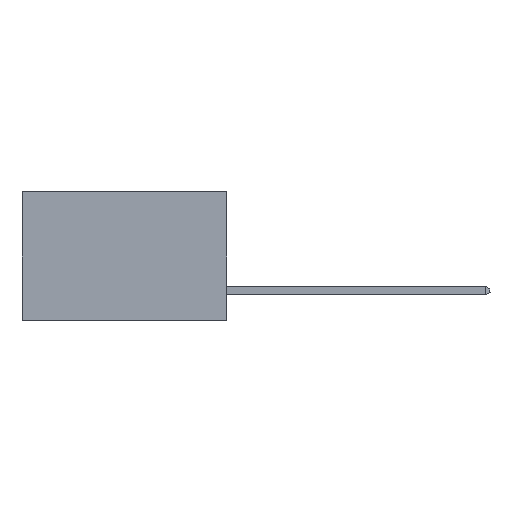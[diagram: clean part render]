
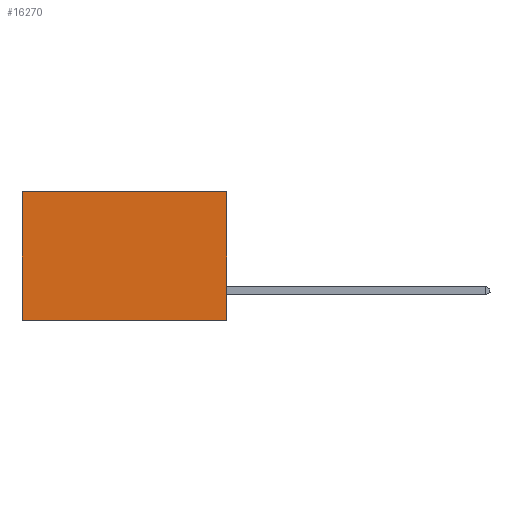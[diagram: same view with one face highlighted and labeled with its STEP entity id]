
A CAD part, left-side view. The second image highlights one B-rep face of the part: STEP entity #16270.
In plain terms, the highlighted planar face has unit normal (-1, 0, 0).
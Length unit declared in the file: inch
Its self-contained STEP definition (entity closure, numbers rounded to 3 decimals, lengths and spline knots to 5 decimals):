
#533 = VERTEX_POINT ( 'NONE', #3240 ) ;
#627 = FACE_OUTER_BOUND ( 'NONE', #21544, .T. ) ;
#714 = EDGE_CURVE ( 'NONE', #16950, #11298, #19438, .T. ) ;
#1269 = DIRECTION ( 'NONE',  ( 0., 0., -1. ) ) ;
#2451 = DIRECTION ( 'NONE',  ( 0., 1., 0. ) ) ;
#3240 = CARTESIAN_POINT ( 'NONE',  ( 0.277, 0.59, 0. ) ) ;
#4111 = CARTESIAN_POINT ( 'NONE',  ( 0.277, 0., -0.37 ) ) ;
#5904 = DIRECTION ( 'NONE',  ( 1., 0., 0. ) ) ;
#6720 = CARTESIAN_POINT ( 'NONE',  ( 0.277, 0., 0. ) ) ;
#7250 = CARTESIAN_POINT ( 'NONE',  ( 0.277, 0., -0.37 ) ) ;
#8171 = ORIENTED_EDGE ( 'NONE', *, *, #14453, .F. ) ;
#9610 = EDGE_CURVE ( 'NONE', #16950, #533, #18718, .T. ) ;
#9711 = CARTESIAN_POINT ( 'NONE',  ( 0.277, 0., -0.37 ) ) ;
#9885 = VECTOR ( 'NONE', #1269, 39.37008 ) ;
#10348 = ORIENTED_EDGE ( 'NONE', *, *, #9610, .T. ) ;
#11298 = VERTEX_POINT ( 'NONE', #15317 ) ;
#12058 = VECTOR ( 'NONE', #2451, 39.37008 ) ;
#12120 = ORIENTED_EDGE ( 'NONE', *, *, #22434, .T. ) ;
#12194 = VECTOR ( 'NONE', #15052, 39.37008 ) ;
#13154 = CARTESIAN_POINT ( 'NONE',  ( 0.277, 0., 0. ) ) ;
#13283 = CARTESIAN_POINT ( 'NONE',  ( 0.277, 0.59, -0.37 ) ) ;
#14453 = EDGE_CURVE ( 'NONE', #11298, #17278, #22154, .T. ) ;
#14880 = PLANE ( 'NONE',  #17425 ) ;
#15052 = DIRECTION ( 'NONE',  ( 0., 0., -1. ) ) ;
#15317 = CARTESIAN_POINT ( 'NONE',  ( 0.277, 0., -0.37 ) ) ;
#16270 = ADVANCED_FACE ( 'NONE', ( #627 ), #14880, .F. ) ;
#16626 = CARTESIAN_POINT ( 'NONE',  ( 0.277, 0.59, -0.37 ) ) ;
#16950 = VERTEX_POINT ( 'NONE', #13154 ) ;
#17278 = VERTEX_POINT ( 'NONE', #16626 ) ;
#17425 = AXIS2_PLACEMENT_3D ( 'NONE', #4111, #5904, #18495 ) ;
#18495 = DIRECTION ( 'NONE',  ( 0., 0., -1. ) ) ;
#18718 = LINE ( 'NONE', #6720, #22942 ) ;
#19438 = LINE ( 'NONE', #7250, #9885 ) ;
#20691 = ORIENTED_EDGE ( 'NONE', *, *, #714, .F. ) ;
#21124 = DIRECTION ( 'NONE',  ( 0., 1., 0. ) ) ;
#21544 = EDGE_LOOP ( 'NONE', ( #12120, #8171, #20691, #10348 ) ) ;
#21742 = LINE ( 'NONE', #13283, #12194 ) ;
#22154 = LINE ( 'NONE', #9711, #12058 ) ;
#22434 = EDGE_CURVE ( 'NONE', #533, #17278, #21742, .T. ) ;
#22942 = VECTOR ( 'NONE', #21124, 39.37008 ) ;
